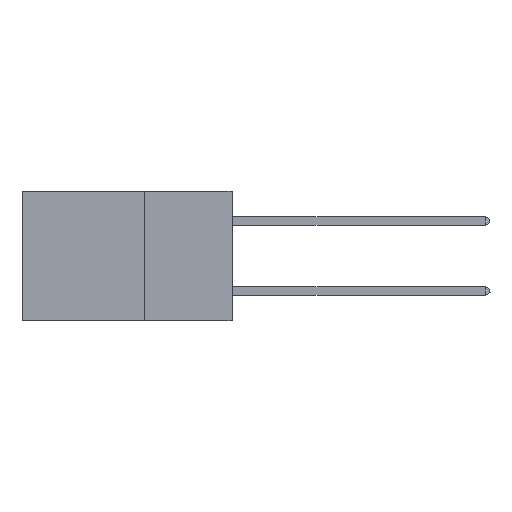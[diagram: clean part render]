
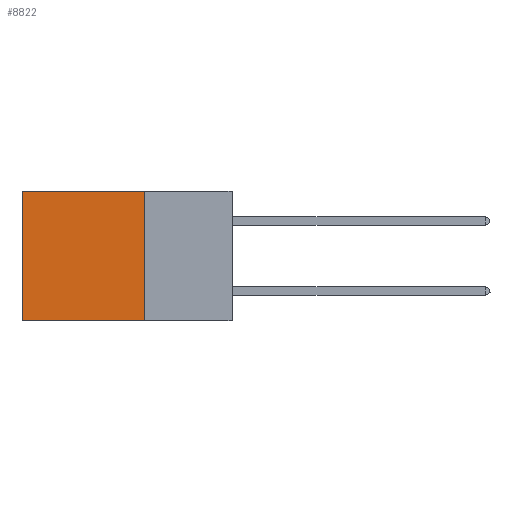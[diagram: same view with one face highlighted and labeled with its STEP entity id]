
A CAD part, left-side view. The second image highlights one B-rep face of the part: STEP entity #8822.
In plain terms, the highlighted planar face has unit normal (-1, 0, 0).
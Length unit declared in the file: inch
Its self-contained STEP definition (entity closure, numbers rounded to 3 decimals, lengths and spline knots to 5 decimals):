
#1328 = LINE ( 'NONE', #25353, #31555 ) ;
#2153 = PLANE ( 'NONE',  #24869 ) ;
#4053 = LINE ( 'NONE', #9739, #10126 ) ;
#4252 = CARTESIAN_POINT ( 'NONE',  ( 0.2875, 0.25, -0.37 ) ) ;
#4832 = CARTESIAN_POINT ( 'NONE',  ( 0.2875, 0.25, -0.37 ) ) ;
#5386 = CARTESIAN_POINT ( 'NONE',  ( 0.2875, 0.25, 0. ) ) ;
#5607 = CARTESIAN_POINT ( 'NONE',  ( 0.2875, 0.6, -0.37 ) ) ;
#6511 = EDGE_CURVE ( 'NONE', #10548, #9172, #29327, .T. ) ;
#7186 = DIRECTION ( 'NONE',  ( 0., 1., 0. ) ) ;
#7455 = EDGE_CURVE ( 'NONE', #30166, #18502, #1328, .T. ) ;
#8210 = DIRECTION ( 'NONE',  ( 0., 0., -1. ) ) ;
#8822 = ADVANCED_FACE ( 'NONE', ( #22660 ), #2153, .F. ) ;
#9098 = EDGE_CURVE ( 'NONE', #30166, #10548, #22418, .T. ) ;
#9172 = VERTEX_POINT ( 'NONE', #5607 ) ;
#9739 = CARTESIAN_POINT ( 'NONE',  ( 0.2875, 0.6, 0. ) ) ;
#9836 = CARTESIAN_POINT ( 'NONE',  ( 0.2875, 0.25, 0. ) ) ;
#10049 = ORIENTED_EDGE ( 'NONE', *, *, #19966, .T. ) ;
#10126 = VECTOR ( 'NONE', #14344, 39.37008 ) ;
#10548 = VERTEX_POINT ( 'NONE', #4252 ) ;
#12061 = DIRECTION ( 'NONE',  ( 0., 0., -1. ) ) ;
#13798 = ORIENTED_EDGE ( 'NONE', *, *, #9098, .F. ) ;
#14344 = DIRECTION ( 'NONE',  ( 0., 0., -1. ) ) ;
#18502 = VERTEX_POINT ( 'NONE', #28663 ) ;
#19345 = ORIENTED_EDGE ( 'NONE', *, *, #6511, .F. ) ;
#19966 = EDGE_CURVE ( 'NONE', #18502, #9172, #4053, .T. ) ;
#21379 = DIRECTION ( 'NONE',  ( 0., 1., 0. ) ) ;
#22418 = LINE ( 'NONE', #5386, #28567 ) ;
#22660 = FACE_OUTER_BOUND ( 'NONE', #26561, .T. ) ;
#24869 = AXIS2_PLACEMENT_3D ( 'NONE', #9836, #31572, #12061 ) ;
#25353 = CARTESIAN_POINT ( 'NONE',  ( 0.2875, 0.25, 0. ) ) ;
#26480 = ORIENTED_EDGE ( 'NONE', *, *, #7455, .T. ) ;
#26561 = EDGE_LOOP ( 'NONE', ( #10049, #19345, #13798, #26480 ) ) ;
#26809 = CARTESIAN_POINT ( 'NONE',  ( 0.2875, 0.25, 0. ) ) ;
#27797 = VECTOR ( 'NONE', #7186, 39.37008 ) ;
#28567 = VECTOR ( 'NONE', #8210, 39.37008 ) ;
#28663 = CARTESIAN_POINT ( 'NONE',  ( 0.2875, 0.6, 0. ) ) ;
#29327 = LINE ( 'NONE', #4832, #27797 ) ;
#30166 = VERTEX_POINT ( 'NONE', #26809 ) ;
#31555 = VECTOR ( 'NONE', #21379, 39.37008 ) ;
#31572 = DIRECTION ( 'NONE',  ( 1., 0., 0. ) ) ;
